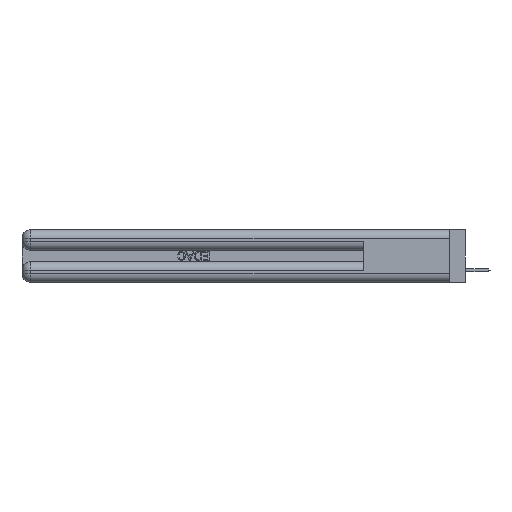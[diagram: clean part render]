
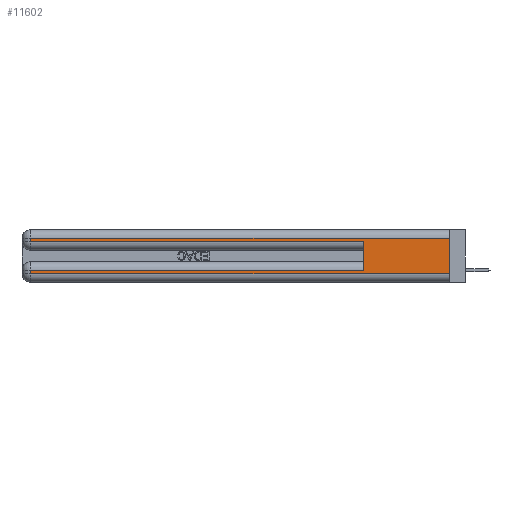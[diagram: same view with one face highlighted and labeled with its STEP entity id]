
A CAD part, left-side view. The second image highlights one B-rep face of the part: STEP entity #11602.
In plain terms, the highlighted planar face has unit normal (-1, 0, 0).
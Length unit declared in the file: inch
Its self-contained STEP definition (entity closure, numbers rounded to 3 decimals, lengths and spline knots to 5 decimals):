
#587 = LINE ( 'NONE', #15878, #31593 ) ;
#1772 = VERTEX_POINT ( 'NONE', #24834 ) ;
#2336 = CARTESIAN_POINT ( 'NONE',  ( 0., 0., 0.31 ) ) ;
#2708 = DIRECTION ( 'NONE',  ( 0., 0., 1. ) ) ;
#2989 = VECTOR ( 'NONE', #21786, 39.37008 ) ;
#3103 = CARTESIAN_POINT ( 'NONE',  ( 0., 2.94, 0.37 ) ) ;
#3326 = EDGE_CURVE ( 'NONE', #16057, #36285, #12180, .T. ) ;
#3461 = VERTEX_POINT ( 'NONE', #4298 ) ;
#4298 = CARTESIAN_POINT ( 'NONE',  ( 0., 0.6, 0.285 ) ) ;
#4501 = EDGE_CURVE ( 'NONE', #1772, #37107, #9155, .T. ) ;
#4564 = CARTESIAN_POINT ( 'NONE',  ( 0., 0., 0.06 ) ) ;
#5669 = VECTOR ( 'NONE', #33938, 39.37008 ) ;
#6075 = CARTESIAN_POINT ( 'NONE',  ( 0., 0., 0.085 ) ) ;
#6724 = FACE_OUTER_BOUND ( 'NONE', #7239, .T. ) ;
#7239 = EDGE_LOOP ( 'NONE', ( #39093, #25438, #38687, #36032, #17952, #19616, #9697, #39692 ) ) ;
#7448 = LINE ( 'NONE', #8062, #27370 ) ;
#8048 = LINE ( 'NONE', #6075, #5669 ) ;
#8062 = CARTESIAN_POINT ( 'NONE',  ( 0., 0., 0.37 ) ) ;
#8440 = VERTEX_POINT ( 'NONE', #4564 ) ;
#9155 = LINE ( 'NONE', #35548, #16462 ) ;
#9231 = AXIS2_PLACEMENT_3D ( 'NONE', #25040, #34600, #18933 ) ;
#9437 = VERTEX_POINT ( 'NONE', #19257 ) ;
#9469 = CARTESIAN_POINT ( 'NONE',  ( 0., 0., 0.06 ) ) ;
#9697 = ORIENTED_EDGE ( 'NONE', *, *, #4501, .T. ) ;
#10598 = EDGE_CURVE ( 'NONE', #36544, #16057, #33964, .T. ) ;
#11602 = ADVANCED_FACE ( 'NONE', ( #6724 ), #37457, .F. ) ;
#12180 = LINE ( 'NONE', #3103, #2989 ) ;
#12342 = DIRECTION ( 'NONE',  ( 0., -1., 0. ) ) ;
#13583 = EDGE_CURVE ( 'NONE', #37107, #8440, #36601, .T. ) ;
#13688 = VECTOR ( 'NONE', #2708, 39.37008 ) ;
#15878 = CARTESIAN_POINT ( 'NONE',  ( 0., 0., 0.285 ) ) ;
#16057 = VERTEX_POINT ( 'NONE', #24934 ) ;
#16462 = VECTOR ( 'NONE', #25843, 39.37008 ) ;
#17952 = ORIENTED_EDGE ( 'NONE', *, *, #18551, .F. ) ;
#18551 = EDGE_CURVE ( 'NONE', #9437, #3461, #39388, .T. ) ;
#18933 = DIRECTION ( 'NONE',  ( 0., 0., -1. ) ) ;
#19257 = CARTESIAN_POINT ( 'NONE',  ( 0., 0.6, 0.085 ) ) ;
#19616 = ORIENTED_EDGE ( 'NONE', *, *, #35734, .T. ) ;
#20819 = DIRECTION ( 'NONE',  ( 0., 0., -1. ) ) ;
#21786 = DIRECTION ( 'NONE',  ( 0., 0., -1. ) ) ;
#22395 = CARTESIAN_POINT ( 'NONE',  ( 0., 2.94, 0.285 ) ) ;
#23626 = CARTESIAN_POINT ( 'NONE',  ( 0., 2.94, 0.06 ) ) ;
#24807 = VECTOR ( 'NONE', #39459, 39.37008 ) ;
#24834 = CARTESIAN_POINT ( 'NONE',  ( 0., 2.94, 0.085 ) ) ;
#24934 = CARTESIAN_POINT ( 'NONE',  ( 0., 2.94, 0.31 ) ) ;
#25040 = CARTESIAN_POINT ( 'NONE',  ( 0., 0., 0.37 ) ) ;
#25438 = ORIENTED_EDGE ( 'NONE', *, *, #10598, .T. ) ;
#25843 = DIRECTION ( 'NONE',  ( 0., 0., -1. ) ) ;
#26311 = EDGE_CURVE ( 'NONE', #36544, #8440, #7448, .T. ) ;
#27198 = EDGE_CURVE ( 'NONE', #36285, #3461, #587, .T. ) ;
#27370 = VECTOR ( 'NONE', #20819, 39.37008 ) ;
#27755 = CARTESIAN_POINT ( 'NONE',  ( 0., 0.6, 0.145 ) ) ;
#31593 = VECTOR ( 'NONE', #37793, 39.37008 ) ;
#33938 = DIRECTION ( 'NONE',  ( 0., 1., 0. ) ) ;
#33964 = LINE ( 'NONE', #36300, #24807 ) ;
#34600 = DIRECTION ( 'NONE',  ( 1., 0., 0. ) ) ;
#35548 = CARTESIAN_POINT ( 'NONE',  ( 0., 2.94, 0.37 ) ) ;
#35734 = EDGE_CURVE ( 'NONE', #9437, #1772, #8048, .T. ) ;
#36032 = ORIENTED_EDGE ( 'NONE', *, *, #27198, .T. ) ;
#36130 = VECTOR ( 'NONE', #12342, 39.37008 ) ;
#36285 = VERTEX_POINT ( 'NONE', #22395 ) ;
#36300 = CARTESIAN_POINT ( 'NONE',  ( 0., 0., 0.31 ) ) ;
#36544 = VERTEX_POINT ( 'NONE', #2336 ) ;
#36601 = LINE ( 'NONE', #9469, #36130 ) ;
#37107 = VERTEX_POINT ( 'NONE', #23626 ) ;
#37457 = PLANE ( 'NONE',  #9231 ) ;
#37793 = DIRECTION ( 'NONE',  ( 0., -1., 0. ) ) ;
#38687 = ORIENTED_EDGE ( 'NONE', *, *, #3326, .T. ) ;
#39093 = ORIENTED_EDGE ( 'NONE', *, *, #26311, .F. ) ;
#39388 = LINE ( 'NONE', #27755, #13688 ) ;
#39459 = DIRECTION ( 'NONE',  ( 0., 1., 0. ) ) ;
#39692 = ORIENTED_EDGE ( 'NONE', *, *, #13583, .T. ) ;
